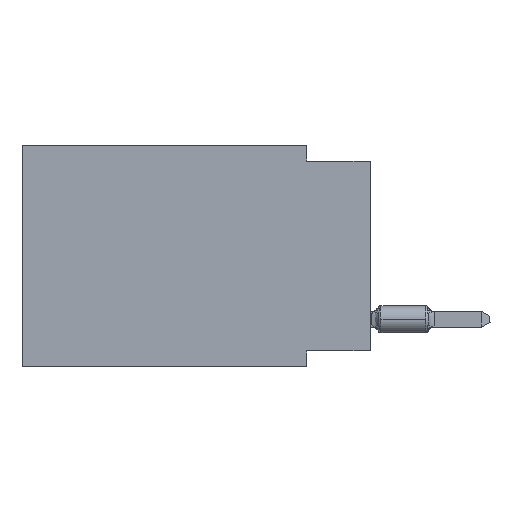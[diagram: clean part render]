
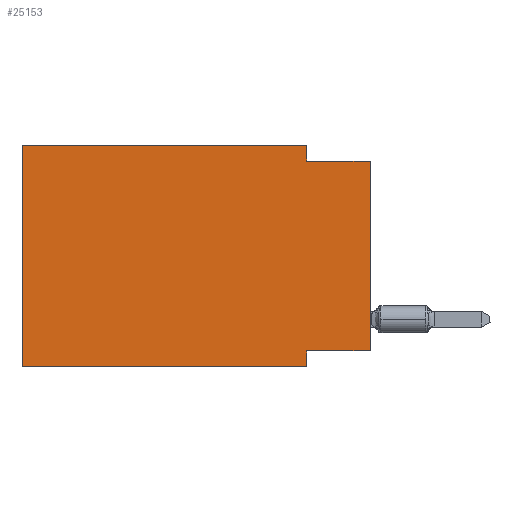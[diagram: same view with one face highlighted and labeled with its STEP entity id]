
A CAD part, left-side view. The second image highlights one B-rep face of the part: STEP entity #25153.
In plain terms, the highlighted planar face has unit normal (-1, 0, 0).
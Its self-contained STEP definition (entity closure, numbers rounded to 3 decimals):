
#238 = VECTOR ( 'NONE', #43142, 1000. ) ;
#520 = DIRECTION ( 'NONE',  ( 0., 0., -1. ) ) ;
#976 = EDGE_CURVE ( 'NONE', #20968, #19402, #13987, .T. ) ;
#1433 = CARTESIAN_POINT ( 'NONE',  ( 0., 13.97, 0. ) ) ;
#1499 = VERTEX_POINT ( 'NONE', #52992 ) ;
#1786 = ORIENTED_EDGE ( 'NONE', *, *, #70527, .F. ) ;
#2703 = DIRECTION ( 'NONE',  ( 0., 1., 0. ) ) ;
#3386 = CARTESIAN_POINT ( 'NONE',  ( 0., 2.54, 0. ) ) ;
#3400 = VERTEX_POINT ( 'NONE', #61563 ) ;
#8805 = LINE ( 'NONE', #64302, #238 ) ;
#8876 = PLANE ( 'NONE',  #10040 ) ;
#9195 = VECTOR ( 'NONE', #520, 1000. ) ;
#9409 = EDGE_CURVE ( 'NONE', #23377, #31827, #49521, .T. ) ;
#9725 = DIRECTION ( 'NONE',  ( 0., 0., 1. ) ) ;
#10040 = AXIS2_PLACEMENT_3D ( 'NONE', #42484, #59264, #65081 ) ;
#10979 = CARTESIAN_POINT ( 'NONE',  ( 0., 2.54, 0. ) ) ;
#12060 = LINE ( 'NONE', #1433, #59688 ) ;
#12400 = CARTESIAN_POINT ( 'NONE',  ( 0., 2.54, -0.635 ) ) ;
#12740 = VERTEX_POINT ( 'NONE', #10979 ) ;
#13987 = LINE ( 'NONE', #36981, #26001 ) ;
#14286 = CARTESIAN_POINT ( 'NONE',  ( 0., 0., -0.635 ) ) ;
#15206 = LINE ( 'NONE', #64506, #32181 ) ;
#19290 = EDGE_CURVE ( 'NONE', #62381, #19402, #8805, .T. ) ;
#19402 = VERTEX_POINT ( 'NONE', #14286 ) ;
#20968 = VERTEX_POINT ( 'NONE', #12400 ) ;
#22792 = CARTESIAN_POINT ( 'NONE',  ( 0., 2.54, -8.89 ) ) ;
#23377 = VERTEX_POINT ( 'NONE', #32923 ) ;
#24303 = EDGE_CURVE ( 'NONE', #3400, #31827, #70448, .T. ) ;
#25153 = ADVANCED_FACE ( 'NONE', ( #53098 ), #8876, .F. ) ;
#26001 = VECTOR ( 'NONE', #31122, 1000. ) ;
#27160 = ORIENTED_EDGE ( 'NONE', *, *, #24303, .T. ) ;
#31122 = DIRECTION ( 'NONE',  ( 0., -1., 0. ) ) ;
#31392 = DIRECTION ( 'NONE',  ( 0., -1., 0. ) ) ;
#31827 = VERTEX_POINT ( 'NONE', #22792 ) ;
#32181 = VECTOR ( 'NONE', #9725, 1000. ) ;
#32923 = CARTESIAN_POINT ( 'NONE',  ( 0., 2.54, -8.255 ) ) ;
#35838 = CARTESIAN_POINT ( 'NONE',  ( 0., 13.97, -8.89 ) ) ;
#36361 = EDGE_LOOP ( 'NONE', ( #48354, #48439, #67876, #39136, #43133, #27160, #48868, #1786 ) ) ;
#36981 = CARTESIAN_POINT ( 'NONE',  ( 0., 0., -0.635 ) ) ;
#37935 = VECTOR ( 'NONE', #31392, 1000. ) ;
#39136 = ORIENTED_EDGE ( 'NONE', *, *, #47817, .F. ) ;
#42484 = CARTESIAN_POINT ( 'NONE',  ( 0., 13.97, 0. ) ) ;
#42490 = LINE ( 'NONE', #3386, #56755 ) ;
#43133 = ORIENTED_EDGE ( 'NONE', *, *, #54864, .F. ) ;
#43142 = DIRECTION ( 'NONE',  ( 0., 0., 1. ) ) ;
#45692 = DIRECTION ( 'NONE',  ( 0., -1., 0. ) ) ;
#46223 = CARTESIAN_POINT ( 'NONE',  ( 0., 0., -8.255 ) ) ;
#47817 = EDGE_CURVE ( 'NONE', #1499, #12740, #12060, .T. ) ;
#48354 = ORIENTED_EDGE ( 'NONE', *, *, #19290, .T. ) ;
#48439 = ORIENTED_EDGE ( 'NONE', *, *, #976, .F. ) ;
#48868 = ORIENTED_EDGE ( 'NONE', *, *, #9409, .F. ) ;
#49521 = LINE ( 'NONE', #67000, #9195 ) ;
#52992 = CARTESIAN_POINT ( 'NONE',  ( 0., 13.97, 0. ) ) ;
#53098 = FACE_OUTER_BOUND ( 'NONE', #36361, .T. ) ;
#54864 = EDGE_CURVE ( 'NONE', #3400, #1499, #15206, .T. ) ;
#55402 = CARTESIAN_POINT ( 'NONE',  ( 0., 0., -8.255 ) ) ;
#56072 = VECTOR ( 'NONE', #2703, 1000. ) ;
#56755 = VECTOR ( 'NONE', #64732, 1000. ) ;
#59264 = DIRECTION ( 'NONE',  ( 1., 0., 0. ) ) ;
#59688 = VECTOR ( 'NONE', #45692, 1000. ) ;
#59692 = EDGE_CURVE ( 'NONE', #12740, #20968, #42490, .T. ) ;
#61563 = CARTESIAN_POINT ( 'NONE',  ( 0., 13.97, -8.89 ) ) ;
#62381 = VERTEX_POINT ( 'NONE', #55402 ) ;
#62642 = LINE ( 'NONE', #46223, #56072 ) ;
#64302 = CARTESIAN_POINT ( 'NONE',  ( 0., 0., 0. ) ) ;
#64506 = CARTESIAN_POINT ( 'NONE',  ( 0., 13.97, 0. ) ) ;
#64732 = DIRECTION ( 'NONE',  ( 0., 0., -1. ) ) ;
#65081 = DIRECTION ( 'NONE',  ( 0., 0., -1. ) ) ;
#67000 = CARTESIAN_POINT ( 'NONE',  ( 0., 2.54, -8.89 ) ) ;
#67876 = ORIENTED_EDGE ( 'NONE', *, *, #59692, .F. ) ;
#70448 = LINE ( 'NONE', #35838, #37935 ) ;
#70527 = EDGE_CURVE ( 'NONE', #62381, #23377, #62642, .T. ) ;
